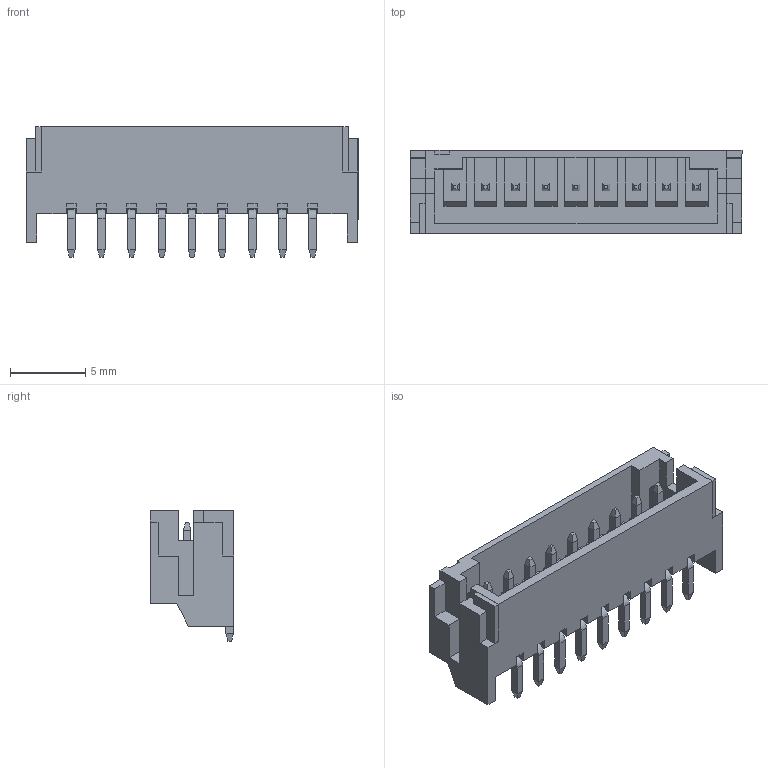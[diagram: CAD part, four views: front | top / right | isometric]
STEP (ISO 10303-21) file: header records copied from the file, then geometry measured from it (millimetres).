
FILE_DESCRIPTION (( 'STEP AP203' ), '1' );
FILE_NAME ('140-509-417-060.STEP', '2020-03-31T20:22:44', ( '' ), ( '' ), 'SwSTEP 2.0', 'SolidWorks 2016', '' );
FILE_SCHEMA (( 'CONFIG_CONTROL_DESIGN' ));
Length unit declared in the file: millimetre
Products named in the file (4): RA SMT Housing_509; RA SMT Contact; RA SMT Pad; 140-509-417-060
Assembly tree (12 placements, depth 2):
  140-509-417-060
    RA SMT Housing_509
    RA SMT Contact  x9
    RA SMT Pad  x2
Bounding box: 22 x 5.5 x 8.65 mm (x, y, z)
Volume: 304.5 mm3; surface area: 1141.8 mm2
Topology: 12 solids, 12 shells, 494 faces, 1204 edges, 730 vertices
Faces by surface type: plane 458, cylinder 36
Entity records: 8662 total; most frequent: CARTESIAN_POINT 1441, ORIENTED_EDGE 1424, DIRECTION 1246, EDGE_CURVE 712, LINE 704, VECTOR 704, VERTEX_POINT 466, AXIS2_PLACEMENT_3D 271
